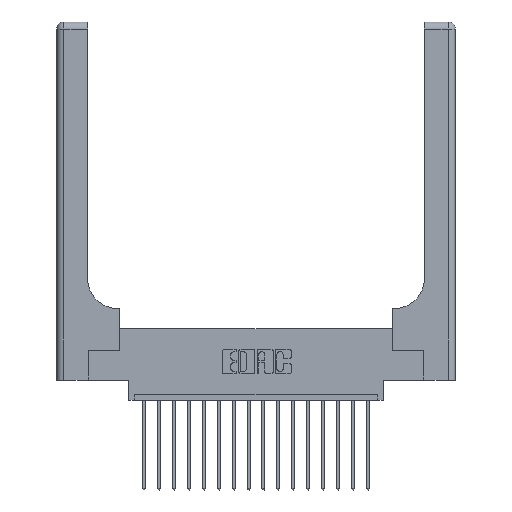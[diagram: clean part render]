
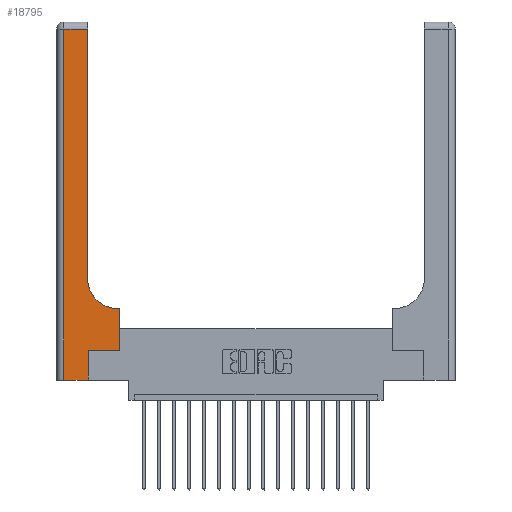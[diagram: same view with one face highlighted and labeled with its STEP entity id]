
A CAD part, top view. The second image highlights one B-rep face of the part: STEP entity #18795.
In plain terms, the highlighted planar face has unit normal (0, 0, 1).
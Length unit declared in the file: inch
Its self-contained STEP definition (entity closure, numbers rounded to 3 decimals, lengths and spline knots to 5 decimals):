
#427 = EDGE_CURVE ( 'NONE', #17257, #11780, #16884, .T. ) ;
#462 = DIRECTION ( 'NONE',  ( 0., 0., -1. ) ) ;
#688 = DIRECTION ( 'NONE',  ( 1., 0., 0. ) ) ;
#1169 = LINE ( 'NONE', #10264, #7708 ) ;
#1565 = EDGE_CURVE ( 'NONE', #8816, #3411, #8697, .T. ) ;
#1843 = CARTESIAN_POINT ( 'NONE',  ( 0.265, 0., 0.37 ) ) ;
#1943 = CARTESIAN_POINT ( 'NONE',  ( 0.26, 0.85, 0.37 ) ) ;
#2130 = VERTEX_POINT ( 'NONE', #7733 ) ;
#2762 = CARTESIAN_POINT ( 'NONE',  ( 0.51, 0.85, 0.37 ) ) ;
#2992 = CARTESIAN_POINT ( 'NONE',  ( 0.528, 0.25, 0.37 ) ) ;
#3045 = DIRECTION ( 'NONE',  ( 1., 0., 0. ) ) ;
#3411 = VERTEX_POINT ( 'NONE', #1943 ) ;
#3480 = VECTOR ( 'NONE', #6238, 39.37008 ) ;
#3499 = EDGE_CURVE ( 'NONE', #14365, #14623, #4367, .T. ) ;
#4165 = CARTESIAN_POINT ( 'NONE',  ( 0.26, 2.94, 0.37 ) ) ;
#4367 = LINE ( 'NONE', #2992, #17934 ) ;
#4480 = EDGE_CURVE ( 'NONE', #11780, #2130, #16595, .T. ) ;
#4764 = ORIENTED_EDGE ( 'NONE', *, *, #427, .T. ) ;
#5053 = FACE_OUTER_BOUND ( 'NONE', #18805, .T. ) ;
#5173 = DIRECTION ( 'NONE',  ( 1., 0., 0. ) ) ;
#5358 = ORIENTED_EDGE ( 'NONE', *, *, #1565, .T. ) ;
#5831 = DIRECTION ( 'NONE',  ( 0., -1., 0. ) ) ;
#6014 = LINE ( 'NONE', #11455, #18977 ) ;
#6238 = DIRECTION ( 'NONE',  ( -1., 0., 0. ) ) ;
#6303 = PLANE ( 'NONE',  #15055 ) ;
#6494 = ORIENTED_EDGE ( 'NONE', *, *, #9305, .T. ) ;
#6728 = ORIENTED_EDGE ( 'NONE', *, *, #4480, .T. ) ;
#6854 = EDGE_CURVE ( 'NONE', #18910, #17257, #1169, .T. ) ;
#7390 = CARTESIAN_POINT ( 'NONE',  ( 0.26, 0.6, 0.37 ) ) ;
#7708 = VECTOR ( 'NONE', #5831, 39.37008 ) ;
#7733 = CARTESIAN_POINT ( 'NONE',  ( 0.265, 0.25, 0.37 ) ) ;
#8270 = CARTESIAN_POINT ( 'NONE',  ( 0.528, 0.25, 0.37 ) ) ;
#8528 = ORIENTED_EDGE ( 'NONE', *, *, #15781, .T. ) ;
#8669 = DIRECTION ( 'NONE',  ( 0., 0., -1. ) ) ;
#8697 = CIRCLE ( 'NONE', #10231, 0.25 ) ;
#8816 = VERTEX_POINT ( 'NONE', #9726 ) ;
#9042 = LINE ( 'NONE', #7390, #3480 ) ;
#9145 = ORIENTED_EDGE ( 'NONE', *, *, #3499, .T. ) ;
#9305 = EDGE_CURVE ( 'NONE', #15220, #18910, #10941, .T. ) ;
#9726 = CARTESIAN_POINT ( 'NONE',  ( 0.51, 0.6, 0.37 ) ) ;
#10000 = VECTOR ( 'NONE', #5173, 39.37008 ) ;
#10231 = AXIS2_PLACEMENT_3D ( 'NONE', #2762, #8669, #3045 ) ;
#10264 = CARTESIAN_POINT ( 'NONE',  ( 0.06, 3., 0.37 ) ) ;
#10712 = ORIENTED_EDGE ( 'NONE', *, *, #12890, .T. ) ;
#10746 = DIRECTION ( 'NONE',  ( 0., 1., 0. ) ) ;
#10828 = DIRECTION ( 'NONE',  ( -1., 0., 0. ) ) ;
#10836 = CARTESIAN_POINT ( 'NONE',  ( 0.265, 0., 0.37 ) ) ;
#10941 = LINE ( 'NONE', #16879, #18868 ) ;
#11238 = EDGE_CURVE ( 'NONE', #14623, #8816, #9042, .T. ) ;
#11455 = CARTESIAN_POINT ( 'NONE',  ( 0.26, 3., 0.37 ) ) ;
#11780 = VERTEX_POINT ( 'NONE', #10836 ) ;
#11794 = CARTESIAN_POINT ( 'NONE',  ( 0.06, 2.94, 0.37 ) ) ;
#12864 = VECTOR ( 'NONE', #688, 39.37008 ) ;
#12890 = EDGE_CURVE ( 'NONE', #3411, #15220, #6014, .T. ) ;
#13666 = CARTESIAN_POINT ( 'NONE',  ( 0., 3., 0.37 ) ) ;
#14365 = VERTEX_POINT ( 'NONE', #8270 ) ;
#14623 = VERTEX_POINT ( 'NONE', #17469 ) ;
#14663 = CARTESIAN_POINT ( 'NONE',  ( 0.06, 0., 0.37 ) ) ;
#15024 = DIRECTION ( 'NONE',  ( 0., 1., 0. ) ) ;
#15055 = AXIS2_PLACEMENT_3D ( 'NONE', #13666, #462, #10828 ) ;
#15220 = VERTEX_POINT ( 'NONE', #4165 ) ;
#15781 = EDGE_CURVE ( 'NONE', #2130, #14365, #16889, .T. ) ;
#16595 = LINE ( 'NONE', #1843, #19143 ) ;
#16788 = CARTESIAN_POINT ( 'NONE',  ( 0.265, 0.25, 0.37 ) ) ;
#16879 = CARTESIAN_POINT ( 'NONE',  ( 0., 2.94, 0.37 ) ) ;
#16884 = LINE ( 'NONE', #18437, #10000 ) ;
#16889 = LINE ( 'NONE', #16788, #12864 ) ;
#17064 = DIRECTION ( 'NONE',  ( -1., 0., 0. ) ) ;
#17257 = VERTEX_POINT ( 'NONE', #14663 ) ;
#17469 = CARTESIAN_POINT ( 'NONE',  ( 0.528, 0.6, 0.37 ) ) ;
#17545 = DIRECTION ( 'NONE',  ( 0., 1., 0. ) ) ;
#17833 = ORIENTED_EDGE ( 'NONE', *, *, #6854, .T. ) ;
#17934 = VECTOR ( 'NONE', #17545, 39.37008 ) ;
#18322 = ORIENTED_EDGE ( 'NONE', *, *, #11238, .T. ) ;
#18437 = CARTESIAN_POINT ( 'NONE',  ( 0., 0., 0.37 ) ) ;
#18795 = ADVANCED_FACE ( 'NONE', ( #5053 ), #6303, .F. ) ;
#18805 = EDGE_LOOP ( 'NONE', ( #10712, #6494, #17833, #4764, #6728, #8528, #9145, #18322, #5358 ) ) ;
#18868 = VECTOR ( 'NONE', #17064, 39.37008 ) ;
#18910 = VERTEX_POINT ( 'NONE', #11794 ) ;
#18977 = VECTOR ( 'NONE', #15024, 39.37008 ) ;
#19143 = VECTOR ( 'NONE', #10746, 39.37008 ) ;
